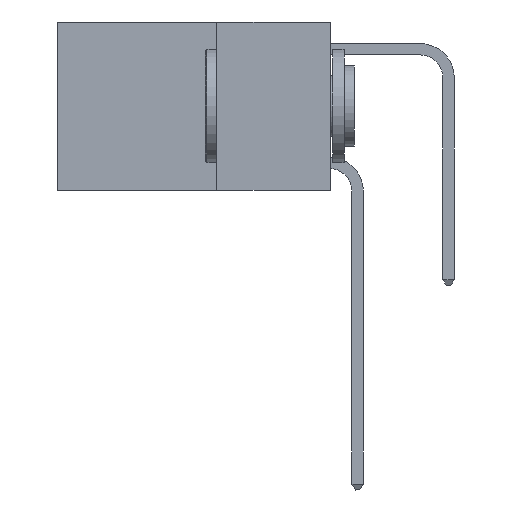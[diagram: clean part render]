
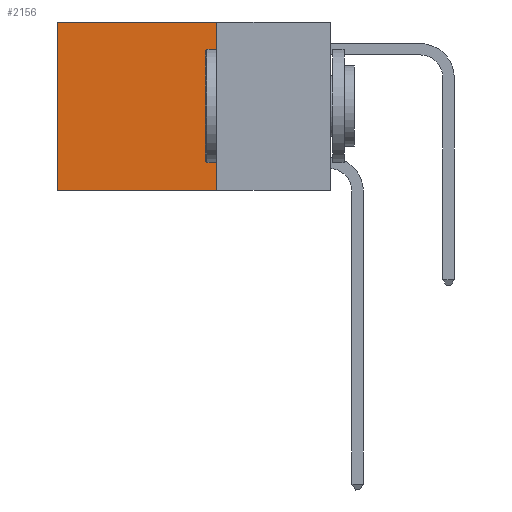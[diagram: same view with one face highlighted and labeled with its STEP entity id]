
A CAD part, left-side view. The second image highlights one B-rep face of the part: STEP entity #2156.
In plain terms, the highlighted planar face has unit normal (-1, 0, 0).
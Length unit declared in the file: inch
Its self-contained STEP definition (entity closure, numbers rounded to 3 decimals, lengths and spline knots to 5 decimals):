
#5 = EDGE_CURVE ( 'NONE', #16988, #17519, #16718, .T. ) ;
#900 = VECTOR ( 'NONE', #11290, 39.37008 ) ;
#1286 = VECTOR ( 'NONE', #8382, 39.37008 ) ;
#2156 = ADVANCED_FACE ( 'NONE', ( #18179 ), #3757, .F. ) ;
#2685 = LINE ( 'NONE', #9115, #15085 ) ;
#3628 = VECTOR ( 'NONE', #6870, 39.37008 ) ;
#3757 = PLANE ( 'NONE',  #18148 ) ;
#4440 = CARTESIAN_POINT ( 'NONE',  ( 0.2625, 0.25, 0. ) ) ;
#6410 = LINE ( 'NONE', #11498, #900 ) ;
#6481 = CARTESIAN_POINT ( 'NONE',  ( 0.2625, 0.6, 0. ) ) ;
#6870 = DIRECTION ( 'NONE',  ( 0., 0., -1. ) ) ;
#6929 = DIRECTION ( 'NONE',  ( 0., 0., -1. ) ) ;
#7610 = ORIENTED_EDGE ( 'NONE', *, *, #9064, .T. ) ;
#7845 = EDGE_LOOP ( 'NONE', ( #11162, #13168, #17257, #7610 ) ) ;
#7886 = VERTEX_POINT ( 'NONE', #19917 ) ;
#8272 = LINE ( 'NONE', #6481, #1286 ) ;
#8302 = CARTESIAN_POINT ( 'NONE',  ( 0.2625, 0.25, -0.37 ) ) ;
#8382 = DIRECTION ( 'NONE',  ( 0., 0., -1. ) ) ;
#9064 = EDGE_CURVE ( 'NONE', #16988, #10764, #2685, .T. ) ;
#9115 = CARTESIAN_POINT ( 'NONE',  ( 0.2625, 0.25, 0. ) ) ;
#9657 = EDGE_CURVE ( 'NONE', #17519, #7886, #6410, .T. ) ;
#10199 = DIRECTION ( 'NONE',  ( 1., 0., 0. ) ) ;
#10399 = DIRECTION ( 'NONE',  ( 0., 1., 0. ) ) ;
#10764 = VERTEX_POINT ( 'NONE', #15161 ) ;
#11162 = ORIENTED_EDGE ( 'NONE', *, *, #14310, .T. ) ;
#11290 = DIRECTION ( 'NONE',  ( 0., 1., 0. ) ) ;
#11498 = CARTESIAN_POINT ( 'NONE',  ( 0.2625, 0.25, -0.37 ) ) ;
#13168 = ORIENTED_EDGE ( 'NONE', *, *, #9657, .F. ) ;
#14310 = EDGE_CURVE ( 'NONE', #10764, #7886, #8272, .T. ) ;
#15085 = VECTOR ( 'NONE', #10399, 39.37008 ) ;
#15161 = CARTESIAN_POINT ( 'NONE',  ( 0.2625, 0.6, 0. ) ) ;
#16718 = LINE ( 'NONE', #18318, #3628 ) ;
#16988 = VERTEX_POINT ( 'NONE', #4440 ) ;
#17257 = ORIENTED_EDGE ( 'NONE', *, *, #5, .F. ) ;
#17519 = VERTEX_POINT ( 'NONE', #8302 ) ;
#18148 = AXIS2_PLACEMENT_3D ( 'NONE', #19986, #10199, #6929 ) ;
#18179 = FACE_OUTER_BOUND ( 'NONE', #7845, .T. ) ;
#18318 = CARTESIAN_POINT ( 'NONE',  ( 0.2625, 0.25, 0. ) ) ;
#19917 = CARTESIAN_POINT ( 'NONE',  ( 0.2625, 0.6, -0.37 ) ) ;
#19986 = CARTESIAN_POINT ( 'NONE',  ( 0.2625, 0.25, 0. ) ) ;
